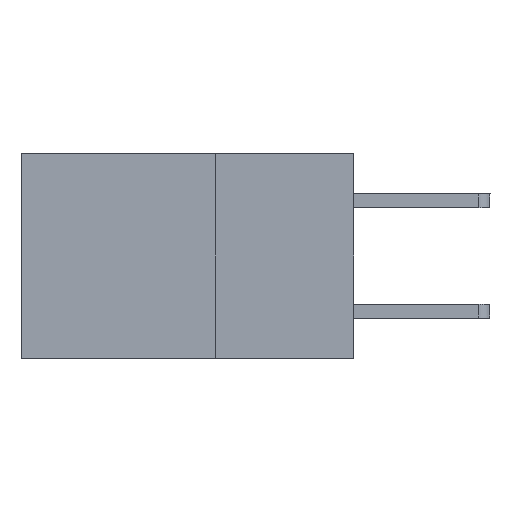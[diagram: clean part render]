
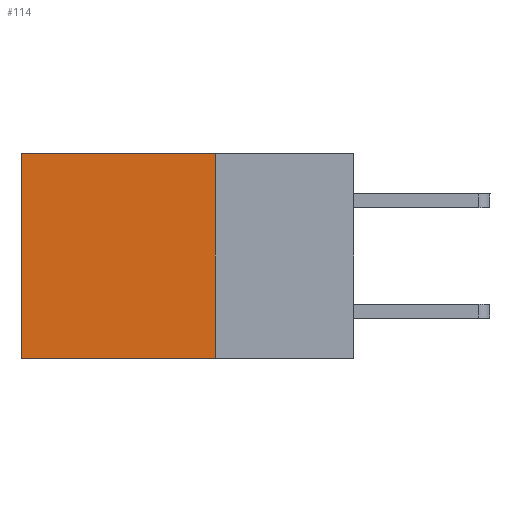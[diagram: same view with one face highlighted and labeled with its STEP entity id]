
A CAD part, left-side view. The second image highlights one B-rep face of the part: STEP entity #114.
In plain terms, the highlighted planar face has unit normal (-1, 0, 0).
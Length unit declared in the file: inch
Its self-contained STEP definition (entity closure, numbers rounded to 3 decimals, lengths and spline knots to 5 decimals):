
#114 = ADVANCED_FACE ( 'NONE', ( #9416 ), #11144, .F. ) ;
#120 = ORIENTED_EDGE ( 'NONE', *, *, #9990, .F. ) ;
#1156 = DIRECTION ( 'NONE',  ( 0., 0., -1. ) ) ;
#1215 = CARTESIAN_POINT ( 'NONE',  ( 0.2875, 0.6, 0. ) ) ;
#1541 = LINE ( 'NONE', #1215, #1905 ) ;
#1731 = ORIENTED_EDGE ( 'NONE', *, *, #2272, .T. ) ;
#1905 = VECTOR ( 'NONE', #1156, 39.37008 ) ;
#2216 = VERTEX_POINT ( 'NONE', #14024 ) ;
#2272 = EDGE_CURVE ( 'NONE', #13620, #8899, #8859, .T. ) ;
#3645 = DIRECTION ( 'NONE',  ( 0., 1., 0. ) ) ;
#3990 = VECTOR ( 'NONE', #3645, 39.37008 ) ;
#4476 = EDGE_CURVE ( 'NONE', #8899, #11047, #1541, .T. ) ;
#5945 = VECTOR ( 'NONE', #11987, 39.37008 ) ;
#6785 = CARTESIAN_POINT ( 'NONE',  ( 0.2875, 0.25, 0. ) ) ;
#6971 = CARTESIAN_POINT ( 'NONE',  ( 0.2875, 0.25, 0. ) ) ;
#7318 = CARTESIAN_POINT ( 'NONE',  ( 0.2875, 0.25, 0. ) ) ;
#7947 = VECTOR ( 'NONE', #10050, 39.37008 ) ;
#8092 = EDGE_LOOP ( 'NONE', ( #8342, #9109, #120, #1731 ) ) ;
#8342 = ORIENTED_EDGE ( 'NONE', *, *, #4476, .T. ) ;
#8563 = CARTESIAN_POINT ( 'NONE',  ( 0.2875, 0.6, -0.37 ) ) ;
#8859 = LINE ( 'NONE', #6971, #5945 ) ;
#8899 = VERTEX_POINT ( 'NONE', #11226 ) ;
#9109 = ORIENTED_EDGE ( 'NONE', *, *, #10075, .F. ) ;
#9416 = FACE_OUTER_BOUND ( 'NONE', #8092, .T. ) ;
#9800 = LINE ( 'NONE', #13282, #3990 ) ;
#9990 = EDGE_CURVE ( 'NONE', #13620, #2216, #10814, .T. ) ;
#10050 = DIRECTION ( 'NONE',  ( 0., 0., -1. ) ) ;
#10075 = EDGE_CURVE ( 'NONE', #2216, #11047, #9800, .T. ) ;
#10097 = AXIS2_PLACEMENT_3D ( 'NONE', #13112, #10164, #12815 ) ;
#10164 = DIRECTION ( 'NONE',  ( 1., 0., 0. ) ) ;
#10814 = LINE ( 'NONE', #6785, #7947 ) ;
#11047 = VERTEX_POINT ( 'NONE', #8563 ) ;
#11144 = PLANE ( 'NONE',  #10097 ) ;
#11226 = CARTESIAN_POINT ( 'NONE',  ( 0.2875, 0.6, 0. ) ) ;
#11987 = DIRECTION ( 'NONE',  ( 0., 1., 0. ) ) ;
#12815 = DIRECTION ( 'NONE',  ( 0., 0., -1. ) ) ;
#13112 = CARTESIAN_POINT ( 'NONE',  ( 0.2875, 0.25, 0. ) ) ;
#13282 = CARTESIAN_POINT ( 'NONE',  ( 0.2875, 0.25, -0.37 ) ) ;
#13620 = VERTEX_POINT ( 'NONE', #7318 ) ;
#14024 = CARTESIAN_POINT ( 'NONE',  ( 0.2875, 0.25, -0.37 ) ) ;
